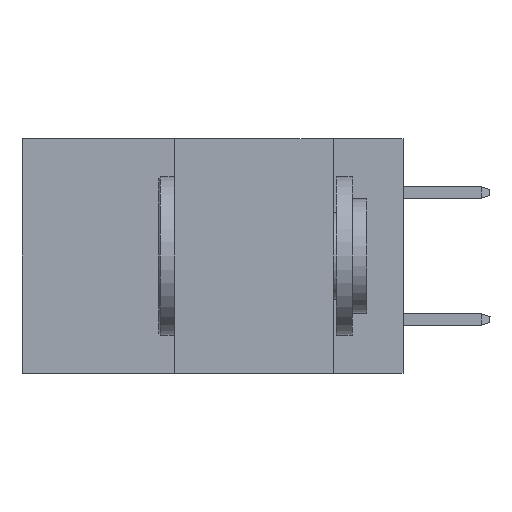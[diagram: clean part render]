
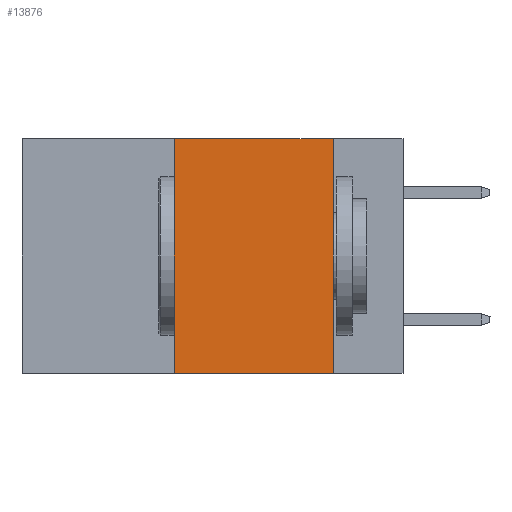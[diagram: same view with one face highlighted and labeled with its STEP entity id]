
A CAD part, left-side view. The second image highlights one B-rep face of the part: STEP entity #13876.
In plain terms, the highlighted planar face has unit normal (-1, 0, 0).
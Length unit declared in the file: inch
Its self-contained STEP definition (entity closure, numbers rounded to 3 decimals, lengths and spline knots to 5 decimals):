
#247 = CARTESIAN_POINT ( 'NONE',  ( 0., 0.6, 0. ) ) ;
#891 = EDGE_CURVE ( 'NONE', #4647, #16655, #21198, .T. ) ;
#1232 = FACE_OUTER_BOUND ( 'NONE', #16555, .T. ) ;
#3026 = CARTESIAN_POINT ( 'NONE',  ( 0., 0.6, -0.37 ) ) ;
#4647 = VERTEX_POINT ( 'NONE', #8365 ) ;
#6653 = LINE ( 'NONE', #18479, #7466 ) ;
#6735 = VECTOR ( 'NONE', #21125, 39.37008 ) ;
#7466 = VECTOR ( 'NONE', #24999, 39.37008 ) ;
#7621 = ORIENTED_EDGE ( 'NONE', *, *, #29800, .F. ) ;
#7859 = EDGE_CURVE ( 'NONE', #11821, #16655, #27966, .T. ) ;
#8191 = DIRECTION ( 'NONE',  ( 0., 0., -1. ) ) ;
#8319 = CARTESIAN_POINT ( 'NONE',  ( 0., 0.36, 0. ) ) ;
#8365 = CARTESIAN_POINT ( 'NONE',  ( 0., 0.36, -0.37 ) ) ;
#11379 = EDGE_CURVE ( 'NONE', #4647, #19910, #6653, .T. ) ;
#11821 = VERTEX_POINT ( 'NONE', #15862 ) ;
#12218 = AXIS2_PLACEMENT_3D ( 'NONE', #14565, #28953, #8191 ) ;
#12522 = ORIENTED_EDGE ( 'NONE', *, *, #11379, .F. ) ;
#13545 = VECTOR ( 'NONE', #14176, 39.37008 ) ;
#13876 = ADVANCED_FACE ( 'NONE', ( #1232 ), #19679, .F. ) ;
#14176 = DIRECTION ( 'NONE',  ( 0., 0., -1. ) ) ;
#14565 = CARTESIAN_POINT ( 'NONE',  ( 0., 0.6, 0. ) ) ;
#14979 = CARTESIAN_POINT ( 'NONE',  ( 0., 0.11, -0.37 ) ) ;
#15862 = CARTESIAN_POINT ( 'NONE',  ( 0., 0.11, 0. ) ) ;
#16555 = EDGE_LOOP ( 'NONE', ( #19955, #7621, #12522, #24187 ) ) ;
#16655 = VERTEX_POINT ( 'NONE', #14979 ) ;
#18479 = CARTESIAN_POINT ( 'NONE',  ( 0., 0.36, 0. ) ) ;
#19679 = PLANE ( 'NONE',  #12218 ) ;
#19910 = VERTEX_POINT ( 'NONE', #8319 ) ;
#19955 = ORIENTED_EDGE ( 'NONE', *, *, #7859, .F. ) ;
#21125 = DIRECTION ( 'NONE',  ( 0., -1., 0. ) ) ;
#21198 = LINE ( 'NONE', #3026, #29802 ) ;
#21356 = DIRECTION ( 'NONE',  ( 0., -1., 0. ) ) ;
#21432 = CARTESIAN_POINT ( 'NONE',  ( 0., 0.11, 0. ) ) ;
#23426 = LINE ( 'NONE', #247, #6735 ) ;
#24187 = ORIENTED_EDGE ( 'NONE', *, *, #891, .T. ) ;
#24999 = DIRECTION ( 'NONE',  ( 0., 0., 1. ) ) ;
#27966 = LINE ( 'NONE', #21432, #13545 ) ;
#28953 = DIRECTION ( 'NONE',  ( 1., 0., 0. ) ) ;
#29800 = EDGE_CURVE ( 'NONE', #19910, #11821, #23426, .T. ) ;
#29802 = VECTOR ( 'NONE', #21356, 39.37008 ) ;
